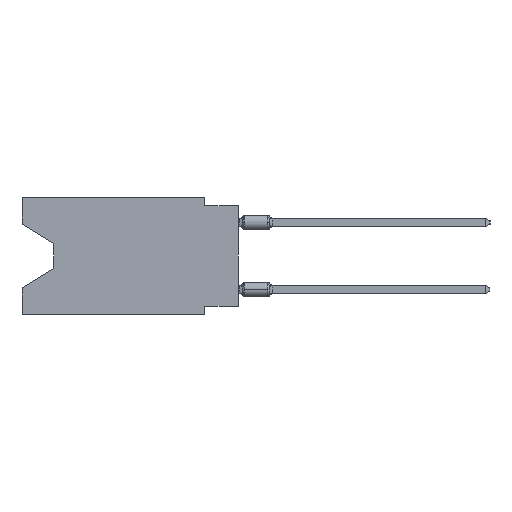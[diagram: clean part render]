
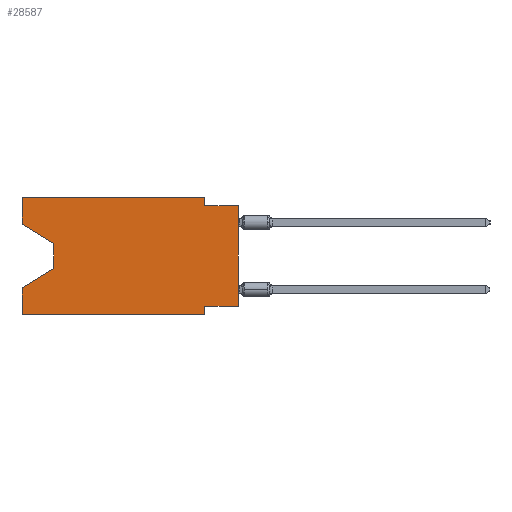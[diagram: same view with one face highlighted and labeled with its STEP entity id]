
A CAD part, left-side view. The second image highlights one B-rep face of the part: STEP entity #28587.
In plain terms, the highlighted planar face has unit normal (-1, 0, 0).
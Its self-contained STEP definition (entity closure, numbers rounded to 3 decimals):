
#77 = EDGE_CURVE ( 'NONE', #26815, #21533, #2711, .T. ) ;
#297 = AXIS2_PLACEMENT_3D ( 'NONE', #3324, #17655, #14928 ) ;
#1471 = VECTOR ( 'NONE', #8798, 1000. ) ;
#2356 = DIRECTION ( 'NONE',  ( 0., 0., 1. ) ) ;
#2571 = ORIENTED_EDGE ( 'NONE', *, *, #38100, .F. ) ;
#2711 = LINE ( 'NONE', #17252, #33722 ) ;
#3324 = CARTESIAN_POINT ( 'NONE',  ( 0., 16.383, 0. ) ) ;
#3425 = EDGE_CURVE ( 'NONE', #21332, #37517, #17269, .T. ) ;
#4539 = EDGE_CURVE ( 'NONE', #26815, #12719, #37226, .T. ) ;
#6496 = EDGE_CURVE ( 'NONE', #34074, #8848, #34560, .T. ) ;
#6559 = LINE ( 'NONE', #27810, #25485 ) ;
#6941 = DIRECTION ( 'NONE',  ( 0., 0., -1. ) ) ;
#7536 = EDGE_CURVE ( 'NONE', #8848, #37517, #21460, .T. ) ;
#7549 = VECTOR ( 'NONE', #16711, 1000. ) ;
#7584 = CARTESIAN_POINT ( 'NONE',  ( 0., 16.383, 0. ) ) ;
#7750 = CARTESIAN_POINT ( 'NONE',  ( 0., 13.97, -3.505 ) ) ;
#8075 = CARTESIAN_POINT ( 'NONE',  ( 0., 16.383, -6.852 ) ) ;
#8389 = LINE ( 'NONE', #35388, #1471 ) ;
#8731 = VECTOR ( 'NONE', #2356, 1000. ) ;
#8798 = DIRECTION ( 'NONE',  ( 0., 0., 1. ) ) ;
#8848 = VERTEX_POINT ( 'NONE', #34070 ) ;
#9007 = FACE_OUTER_BOUND ( 'NONE', #23878, .T. ) ;
#9020 = DIRECTION ( 'NONE',  ( 0., -1., 0. ) ) ;
#9669 = EDGE_CURVE ( 'NONE', #21332, #19643, #21828, .T. ) ;
#10414 = EDGE_CURVE ( 'NONE', #12719, #19643, #11831, .T. ) ;
#10725 = VECTOR ( 'NONE', #15172, 1000. ) ;
#11831 = LINE ( 'NONE', #23833, #34256 ) ;
#12719 = VERTEX_POINT ( 'NONE', #37803 ) ;
#13201 = ORIENTED_EDGE ( 'NONE', *, *, #15260, .T. ) ;
#14619 = VERTEX_POINT ( 'NONE', #23674 ) ;
#14715 = ORIENTED_EDGE ( 'NONE', *, *, #6496, .T. ) ;
#14928 = DIRECTION ( 'NONE',  ( 0., 0., -1. ) ) ;
#15172 = DIRECTION ( 'NONE',  ( 0., 0.855, -0.519 ) ) ;
#15260 = EDGE_CURVE ( 'NONE', #38372, #34074, #23232, .T. ) ;
#15806 = CARTESIAN_POINT ( 'NONE',  ( 0., 0., -8.255 ) ) ;
#16485 = ORIENTED_EDGE ( 'NONE', *, *, #4539, .F. ) ;
#16711 = DIRECTION ( 'NONE',  ( 0., 1., 0. ) ) ;
#17041 = ORIENTED_EDGE ( 'NONE', *, *, #10414, .F. ) ;
#17252 = CARTESIAN_POINT ( 'NONE',  ( 0., 0., 0. ) ) ;
#17269 = LINE ( 'NONE', #29287, #8731 ) ;
#17655 = DIRECTION ( 'NONE',  ( 1., 0., 0. ) ) ;
#18826 = DIRECTION ( 'NONE',  ( 0., -1., 0. ) ) ;
#19287 = VECTOR ( 'NONE', #18826, 1000. ) ;
#19464 = VECTOR ( 'NONE', #31008, 1000. ) ;
#19643 = VERTEX_POINT ( 'NONE', #38370 ) ;
#19654 = CARTESIAN_POINT ( 'NONE',  ( 0., 0., -8.255 ) ) ;
#19953 = EDGE_CURVE ( 'NONE', #35156, #33085, #23136, .T. ) ;
#20474 = DIRECTION ( 'NONE',  ( 0., -0.855, -0.519 ) ) ;
#20755 = ORIENTED_EDGE ( 'NONE', *, *, #31286, .F. ) ;
#20810 = ORIENTED_EDGE ( 'NONE', *, *, #19953, .F. ) ;
#21332 = VERTEX_POINT ( 'NONE', #23084 ) ;
#21407 = PLANE ( 'NONE',  #297 ) ;
#21460 = LINE ( 'NONE', #33680, #10725 ) ;
#21533 = VERTEX_POINT ( 'NONE', #36499 ) ;
#21828 = LINE ( 'NONE', #33245, #23487 ) ;
#21937 = CARTESIAN_POINT ( 'NONE',  ( 0., 16.383, -2.038 ) ) ;
#22582 = ORIENTED_EDGE ( 'NONE', *, *, #3425, .F. ) ;
#23084 = CARTESIAN_POINT ( 'NONE',  ( 0., 16.383, -8.89 ) ) ;
#23136 = LINE ( 'NONE', #7584, #35098 ) ;
#23232 = LINE ( 'NONE', #35856, #32208 ) ;
#23259 = CARTESIAN_POINT ( 'NONE',  ( 0., 16.383, 0. ) ) ;
#23351 = DIRECTION ( 'NONE',  ( 0., 0., 1. ) ) ;
#23487 = VECTOR ( 'NONE', #9020, 1000. ) ;
#23674 = CARTESIAN_POINT ( 'NONE',  ( 0., 2.54, -0.635 ) ) ;
#23833 = CARTESIAN_POINT ( 'NONE',  ( 0., 2.54, -8.89 ) ) ;
#23878 = EDGE_LOOP ( 'NONE', ( #13201, #14715, #36443, #22582, #23972, #17041, #16485, #24294, #35215, #20755, #20810, #2571 ) ) ;
#23972 = ORIENTED_EDGE ( 'NONE', *, *, #9669, .T. ) ;
#24294 = ORIENTED_EDGE ( 'NONE', *, *, #77, .T. ) ;
#24706 = EDGE_CURVE ( 'NONE', #14619, #21533, #31228, .T. ) ;
#24831 = CARTESIAN_POINT ( 'NONE',  ( 0., 13.97, -3.505 ) ) ;
#25485 = VECTOR ( 'NONE', #6941, 1000. ) ;
#26815 = VERTEX_POINT ( 'NONE', #15806 ) ;
#27681 = CARTESIAN_POINT ( 'NONE',  ( 0., 0., -0.635 ) ) ;
#27810 = CARTESIAN_POINT ( 'NONE',  ( 0., 2.54, 0. ) ) ;
#28587 = ADVANCED_FACE ( 'NONE', ( #9007 ), #21407, .F. ) ;
#29287 = CARTESIAN_POINT ( 'NONE',  ( 0., 16.383, 0. ) ) ;
#31008 = DIRECTION ( 'NONE',  ( 0., 0., -1. ) ) ;
#31228 = LINE ( 'NONE', #27681, #19287 ) ;
#31286 = EDGE_CURVE ( 'NONE', #33085, #14619, #6559, .T. ) ;
#31586 = CARTESIAN_POINT ( 'NONE',  ( 0., 2.54, 0. ) ) ;
#31809 = DIRECTION ( 'NONE',  ( 0., -1., 0. ) ) ;
#32208 = VECTOR ( 'NONE', #20474, 1000. ) ;
#33085 = VERTEX_POINT ( 'NONE', #31586 ) ;
#33245 = CARTESIAN_POINT ( 'NONE',  ( 0., 16.383, -8.89 ) ) ;
#33680 = CARTESIAN_POINT ( 'NONE',  ( 0., 13.97, -5.385 ) ) ;
#33722 = VECTOR ( 'NONE', #23351, 1000. ) ;
#34070 = CARTESIAN_POINT ( 'NONE',  ( 0., 13.97, -5.385 ) ) ;
#34074 = VERTEX_POINT ( 'NONE', #24831 ) ;
#34256 = VECTOR ( 'NONE', #38441, 1000. ) ;
#34560 = LINE ( 'NONE', #7750, #19464 ) ;
#35098 = VECTOR ( 'NONE', #31809, 1000. ) ;
#35156 = VERTEX_POINT ( 'NONE', #23259 ) ;
#35215 = ORIENTED_EDGE ( 'NONE', *, *, #24706, .F. ) ;
#35388 = CARTESIAN_POINT ( 'NONE',  ( 0., 16.383, 0. ) ) ;
#35856 = CARTESIAN_POINT ( 'NONE',  ( 0., 16.383, -2.038 ) ) ;
#36443 = ORIENTED_EDGE ( 'NONE', *, *, #7536, .T. ) ;
#36499 = CARTESIAN_POINT ( 'NONE',  ( 0., 0., -0.635 ) ) ;
#37226 = LINE ( 'NONE', #19654, #7549 ) ;
#37517 = VERTEX_POINT ( 'NONE', #8075 ) ;
#37803 = CARTESIAN_POINT ( 'NONE',  ( 0., 2.54, -8.255 ) ) ;
#38100 = EDGE_CURVE ( 'NONE', #38372, #35156, #8389, .T. ) ;
#38370 = CARTESIAN_POINT ( 'NONE',  ( 0., 2.54, -8.89 ) ) ;
#38372 = VERTEX_POINT ( 'NONE', #21937 ) ;
#38441 = DIRECTION ( 'NONE',  ( 0., 0., -1. ) ) ;
